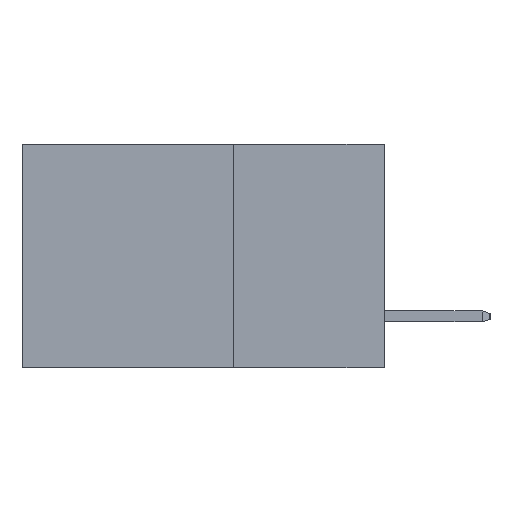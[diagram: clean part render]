
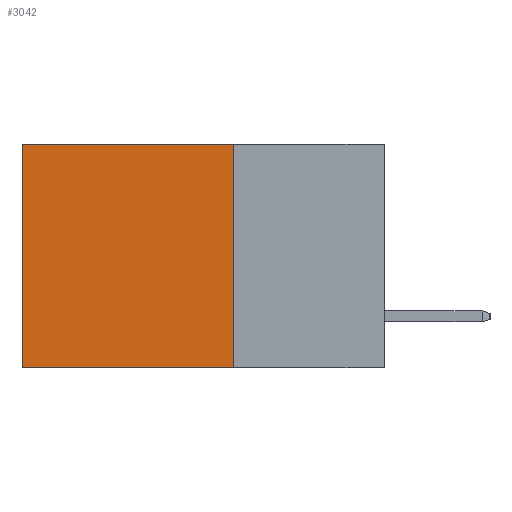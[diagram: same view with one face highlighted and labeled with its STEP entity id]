
A CAD part, left-side view. The second image highlights one B-rep face of the part: STEP entity #3042.
In plain terms, the highlighted planar face has unit normal (-1, 0, 0).
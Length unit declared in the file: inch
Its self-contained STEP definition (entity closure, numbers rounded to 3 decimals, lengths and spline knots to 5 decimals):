
#198 = CARTESIAN_POINT ( 'NONE',  ( 0.298, 0.25, -0.37 ) ) ;
#473 = LINE ( 'NONE', #198, #10158 ) ;
#552 = VECTOR ( 'NONE', #10274, 39.37008 ) ;
#1811 = CARTESIAN_POINT ( 'NONE',  ( 0.298, 0.25, 0. ) ) ;
#2215 = PLANE ( 'NONE',  #12477 ) ;
#2260 = DIRECTION ( 'NONE',  ( 1., 0., 0. ) ) ;
#2670 = EDGE_CURVE ( 'NONE', #13326, #15235, #4532, .T. ) ;
#2694 = DIRECTION ( 'NONE',  ( 0., 0., -1. ) ) ;
#3042 = ADVANCED_FACE ( 'NONE', ( #11649 ), #2215, .F. ) ;
#3148 = ORIENTED_EDGE ( 'NONE', *, *, #14611, .F. ) ;
#3819 = LINE ( 'NONE', #14440, #12971 ) ;
#4532 = LINE ( 'NONE', #10329, #552 ) ;
#5389 = LINE ( 'NONE', #13639, #11731 ) ;
#5467 = DIRECTION ( 'NONE',  ( 0., 1., 0. ) ) ;
#7051 = CARTESIAN_POINT ( 'NONE',  ( 0.298, 0.25, -0.37 ) ) ;
#7721 = CARTESIAN_POINT ( 'NONE',  ( 0.298, 0.6, -0.37 ) ) ;
#8589 = DIRECTION ( 'NONE',  ( 0., 0., -1. ) ) ;
#8965 = DIRECTION ( 'NONE',  ( 0., 1., 0. ) ) ;
#9905 = CARTESIAN_POINT ( 'NONE',  ( 0.298, 0.6, 0. ) ) ;
#10158 = VECTOR ( 'NONE', #5467, 39.37008 ) ;
#10186 = CARTESIAN_POINT ( 'NONE',  ( 0.298, 0.25, 0. ) ) ;
#10274 = DIRECTION ( 'NONE',  ( 0., 0., -1. ) ) ;
#10329 = CARTESIAN_POINT ( 'NONE',  ( 0.298, 0.25, 0. ) ) ;
#10843 = VERTEX_POINT ( 'NONE', #7721 ) ;
#11349 = EDGE_CURVE ( 'NONE', #13326, #15066, #5389, .T. ) ;
#11649 = FACE_OUTER_BOUND ( 'NONE', #14127, .T. ) ;
#11731 = VECTOR ( 'NONE', #8965, 39.37008 ) ;
#12477 = AXIS2_PLACEMENT_3D ( 'NONE', #1811, #2260, #2694 ) ;
#12971 = VECTOR ( 'NONE', #8589, 39.37008 ) ;
#13100 = EDGE_CURVE ( 'NONE', #15066, #10843, #3819, .T. ) ;
#13209 = ORIENTED_EDGE ( 'NONE', *, *, #11349, .T. ) ;
#13326 = VERTEX_POINT ( 'NONE', #10186 ) ;
#13335 = ORIENTED_EDGE ( 'NONE', *, *, #13100, .T. ) ;
#13639 = CARTESIAN_POINT ( 'NONE',  ( 0.298, 0.25, 0. ) ) ;
#14127 = EDGE_LOOP ( 'NONE', ( #13335, #3148, #14658, #13209 ) ) ;
#14440 = CARTESIAN_POINT ( 'NONE',  ( 0.298, 0.6, 0. ) ) ;
#14611 = EDGE_CURVE ( 'NONE', #15235, #10843, #473, .T. ) ;
#14658 = ORIENTED_EDGE ( 'NONE', *, *, #2670, .F. ) ;
#15066 = VERTEX_POINT ( 'NONE', #9905 ) ;
#15235 = VERTEX_POINT ( 'NONE', #7051 ) ;
